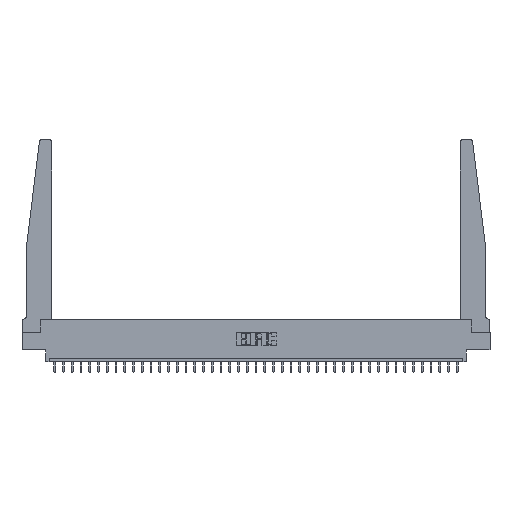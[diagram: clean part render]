
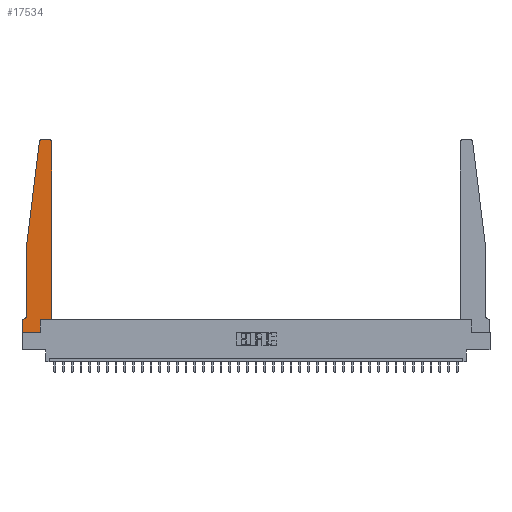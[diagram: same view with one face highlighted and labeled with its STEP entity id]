
A CAD part, top view. The second image highlights one B-rep face of the part: STEP entity #17534.
In plain terms, the highlighted planar face has unit normal (0, 0, 1).
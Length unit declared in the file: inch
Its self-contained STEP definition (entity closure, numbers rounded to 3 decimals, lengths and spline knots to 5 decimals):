
#182 = VERTEX_POINT ( 'NONE', #17547 ) ;
#233 = EDGE_CURVE ( 'NONE', #11087, #182, #4336, .T. ) ;
#707 = DIRECTION ( 'NONE',  ( -1., 0., 0. ) ) ;
#936 = CARTESIAN_POINT ( 'NONE',  ( 0., 0.1875, 0.37 ) ) ;
#964 = CARTESIAN_POINT ( 'NONE',  ( 0.065, 1.25, 0.37 ) ) ;
#1371 = DIRECTION ( 'NONE',  ( 1., 0., 0. ) ) ;
#1618 = LINE ( 'NONE', #12063, #16856 ) ;
#1690 = LINE ( 'NONE', #22586, #21953 ) ;
#1791 = DIRECTION ( 'NONE',  ( 0., 0., 1. ) ) ;
#3959 = CARTESIAN_POINT ( 'NONE',  ( 0.25, 2.75, 0.37 ) ) ;
#4310 = EDGE_CURVE ( 'NONE', #9786, #9453, #16605, .T. ) ;
#4336 = CIRCLE ( 'NONE', #11980, 0.05 ) ;
#6028 = VERTEX_POINT ( 'NONE', #13998 ) ;
#6183 = EDGE_CURVE ( 'NONE', #6589, #31270, #17956, .T. ) ;
#6510 = CARTESIAN_POINT ( 'NONE',  ( 0.425, 0.18, 0.37 ) ) ;
#6589 = VERTEX_POINT ( 'NONE', #20482 ) ;
#7407 = CARTESIAN_POINT ( 'NONE',  ( 0., 0., 0.37 ) ) ;
#8006 = CARTESIAN_POINT ( 'NONE',  ( 0.425, 0.18, 0.37 ) ) ;
#8476 = AXIS2_PLACEMENT_3D ( 'NONE', #27996, #1791, #25594 ) ;
#8853 = ORIENTED_EDGE ( 'NONE', *, *, #233, .T. ) ;
#9453 = VERTEX_POINT ( 'NONE', #8006 ) ;
#9786 = VERTEX_POINT ( 'NONE', #18587 ) ;
#9921 = VERTEX_POINT ( 'NONE', #936 ) ;
#10164 = EDGE_LOOP ( 'NONE', ( #26660, #26125, #26997, #19750, #8853, #19455, #22135, #31441, #10539, #18138, #19765, #17912 ) ) ;
#10539 = ORIENTED_EDGE ( 'NONE', *, *, #23981, .T. ) ;
#10613 = CARTESIAN_POINT ( 'NONE',  ( 0.24675, 2.72367, 0.37 ) ) ;
#10977 = LINE ( 'NONE', #19029, #16732 ) ;
#11087 = VERTEX_POINT ( 'NONE', #13616 ) ;
#11162 = DIRECTION ( 'NONE',  ( 0., 0., -1. ) ) ;
#11552 = VECTOR ( 'NONE', #28827, 39.37008 ) ;
#11746 = CARTESIAN_POINT ( 'NONE',  ( 0.395, 2.75, 0.37 ) ) ;
#11967 = EDGE_CURVE ( 'NONE', #9921, #26111, #15797, .T. ) ;
#11980 = AXIS2_PLACEMENT_3D ( 'NONE', #18539, #11162, #21609 ) ;
#12063 = CARTESIAN_POINT ( 'NONE',  ( 0., 0., 0.37 ) ) ;
#12277 = CARTESIAN_POINT ( 'NONE',  ( 0.425, 0.18, 0.37 ) ) ;
#12303 = DIRECTION ( 'NONE',  ( 0., 0., 1. ) ) ;
#12444 = DIRECTION ( 'NONE',  ( 0., 1., 0. ) ) ;
#13424 = PLANE ( 'NONE',  #32110 ) ;
#13616 = CARTESIAN_POINT ( 'NONE',  ( 0.065, 0.2375, 0.37 ) ) ;
#13998 = CARTESIAN_POINT ( 'NONE',  ( 0.2605, 0., 0.37 ) ) ;
#14664 = LINE ( 'NONE', #12277, #16127 ) ;
#14694 = DIRECTION ( 'NONE',  ( 1., 0., 0. ) ) ;
#15476 = VECTOR ( 'NONE', #29724, 39.37008 ) ;
#15797 = LINE ( 'NONE', #18367, #11552 ) ;
#15907 = CARTESIAN_POINT ( 'NONE',  ( 0.065, 1.25, 0.37 ) ) ;
#16127 = VECTOR ( 'NONE', #12444, 39.37008 ) ;
#16177 = EDGE_CURVE ( 'NONE', #182, #9921, #10977, .T. ) ;
#16189 = CARTESIAN_POINT ( 'NONE',  ( 0.065, 1.25, 0.37 ) ) ;
#16219 = CARTESIAN_POINT ( 'NONE',  ( 0.425, 2.72, 0.37 ) ) ;
#16496 = DIRECTION ( 'NONE',  ( 1., 0., 0. ) ) ;
#16605 = LINE ( 'NONE', #6510, #29295 ) ;
#16732 = VECTOR ( 'NONE', #707, 39.37008 ) ;
#16856 = VECTOR ( 'NONE', #22520, 39.37008 ) ;
#17080 = VECTOR ( 'NONE', #26365, 39.37008 ) ;
#17534 = ADVANCED_FACE ( 'NONE', ( #21313 ), #13424, .T. ) ;
#17547 = CARTESIAN_POINT ( 'NONE',  ( 0.015, 0.1875, 0.37 ) ) ;
#17912 = ORIENTED_EDGE ( 'NONE', *, *, #30628, .T. ) ;
#17956 = CIRCLE ( 'NONE', #25621, 0.03 ) ;
#18138 = ORIENTED_EDGE ( 'NONE', *, *, #4310, .T. ) ;
#18367 = CARTESIAN_POINT ( 'NONE',  ( 0., 0., 0.37 ) ) ;
#18378 = VERTEX_POINT ( 'NONE', #964 ) ;
#18539 = CARTESIAN_POINT ( 'NONE',  ( 0.015, 0.2375, 0.37 ) ) ;
#18587 = CARTESIAN_POINT ( 'NONE',  ( 0.2605, 0.18, 0.37 ) ) ;
#18931 = EDGE_CURVE ( 'NONE', #26111, #6028, #1618, .T. ) ;
#19029 = CARTESIAN_POINT ( 'NONE',  ( 0.065, 0.1875, 0.37 ) ) ;
#19455 = ORIENTED_EDGE ( 'NONE', *, *, #16177, .T. ) ;
#19750 = ORIENTED_EDGE ( 'NONE', *, *, #25325, .T. ) ;
#19765 = ORIENTED_EDGE ( 'NONE', *, *, #30198, .T. ) ;
#19856 = EDGE_CURVE ( 'NONE', #22116, #6589, #27415, .T. ) ;
#20482 = CARTESIAN_POINT ( 'NONE',  ( 0.27653, 2.75, 0.37 ) ) ;
#21313 = FACE_OUTER_BOUND ( 'NONE', #10164, .T. ) ;
#21609 = DIRECTION ( 'NONE',  ( -1., 0., 0. ) ) ;
#21953 = VECTOR ( 'NONE', #30440, 39.37008 ) ;
#22116 = VERTEX_POINT ( 'NONE', #11746 ) ;
#22135 = ORIENTED_EDGE ( 'NONE', *, *, #11967, .T. ) ;
#22520 = DIRECTION ( 'NONE',  ( 1., 0., 0. ) ) ;
#22586 = CARTESIAN_POINT ( 'NONE',  ( 0.2605, 0.18, 0.37 ) ) ;
#22589 = CARTESIAN_POINT ( 'NONE',  ( 0.27653, 2.72, 0.37 ) ) ;
#23886 = DIRECTION ( 'NONE',  ( 0., 0., 1. ) ) ;
#23981 = EDGE_CURVE ( 'NONE', #6028, #9786, #1690, .T. ) ;
#24501 = DIRECTION ( 'NONE',  ( -1., 0., 0. ) ) ;
#25325 = EDGE_CURVE ( 'NONE', #18378, #11087, #31330, .T. ) ;
#25594 = DIRECTION ( 'NONE',  ( 1., 0., 0. ) ) ;
#25621 = AXIS2_PLACEMENT_3D ( 'NONE', #22589, #12303, #14694 ) ;
#26111 = VERTEX_POINT ( 'NONE', #7407 ) ;
#26125 = ORIENTED_EDGE ( 'NONE', *, *, #6183, .T. ) ;
#26365 = DIRECTION ( 'NONE',  ( 0., -1., 0. ) ) ;
#26660 = ORIENTED_EDGE ( 'NONE', *, *, #19856, .T. ) ;
#26665 = VECTOR ( 'NONE', #24501, 39.37008 ) ;
#26997 = ORIENTED_EDGE ( 'NONE', *, *, #27300, .T. ) ;
#27300 = EDGE_CURVE ( 'NONE', #31270, #18378, #31951, .T. ) ;
#27415 = LINE ( 'NONE', #3959, #26665 ) ;
#27996 = CARTESIAN_POINT ( 'NONE',  ( 0.395, 2.72, 0.37 ) ) ;
#28827 = DIRECTION ( 'NONE',  ( 0., -1., 0. ) ) ;
#29295 = VECTOR ( 'NONE', #1371, 39.37008 ) ;
#29724 = DIRECTION ( 'NONE',  ( -0.122, -0.992, 0. ) ) ;
#30198 = EDGE_CURVE ( 'NONE', #9453, #31965, #14664, .T. ) ;
#30440 = DIRECTION ( 'NONE',  ( 0., 1., 0. ) ) ;
#30628 = EDGE_CURVE ( 'NONE', #31965, #22116, #31997, .T. ) ;
#31270 = VERTEX_POINT ( 'NONE', #10613 ) ;
#31330 = LINE ( 'NONE', #15907, #17080 ) ;
#31441 = ORIENTED_EDGE ( 'NONE', *, *, #18931, .T. ) ;
#31951 = LINE ( 'NONE', #16189, #15476 ) ;
#31965 = VERTEX_POINT ( 'NONE', #16219 ) ;
#31997 = CIRCLE ( 'NONE', #8476, 0.03 ) ;
#32084 = CARTESIAN_POINT ( 'NONE',  ( 0., 0.1875, 0.37 ) ) ;
#32110 = AXIS2_PLACEMENT_3D ( 'NONE', #32084, #23886, #16496 ) ;
